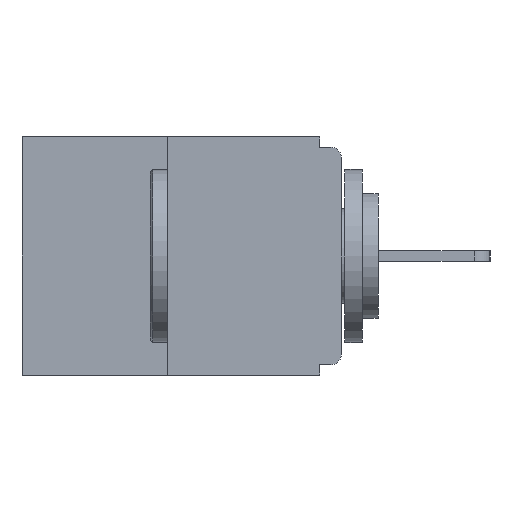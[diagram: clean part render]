
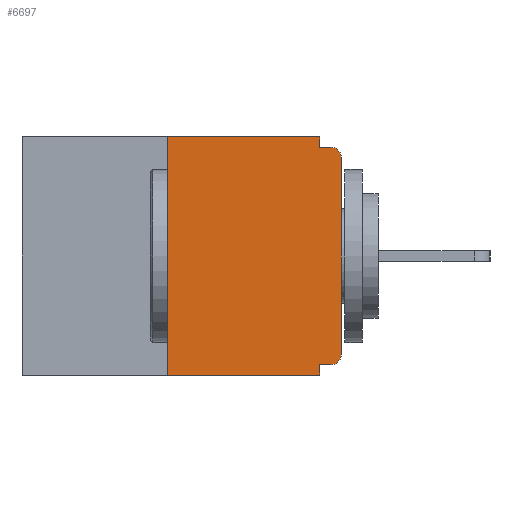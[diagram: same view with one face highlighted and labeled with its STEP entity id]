
A CAD part, left-side view. The second image highlights one B-rep face of the part: STEP entity #6697.
In plain terms, the highlighted planar face has unit normal (-1, 0, 0).
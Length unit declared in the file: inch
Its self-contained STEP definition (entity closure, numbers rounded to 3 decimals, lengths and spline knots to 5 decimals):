
#304 = DIRECTION ( 'NONE',  ( 0., 0., -1. ) ) ;
#586 = VERTEX_POINT ( 'NONE', #8508 ) ;
#661 = CARTESIAN_POINT ( 'NONE',  ( 0., 0.015, -0.015 ) ) ;
#724 = ORIENTED_EDGE ( 'NONE', *, *, #22396, .F. ) ;
#886 = DIRECTION ( 'NONE',  ( 0., -1., 0. ) ) ;
#901 = AXIS2_PLACEMENT_3D ( 'NONE', #9115, #12969, #13385 ) ;
#1353 = LINE ( 'NONE', #16869, #15853 ) ;
#2027 = LINE ( 'NONE', #10971, #6311 ) ;
#2299 = CARTESIAN_POINT ( 'NONE',  ( 0., 0.25, -0.343 ) ) ;
#2434 = EDGE_CURVE ( 'NONE', #12994, #24758, #2027, .T. ) ;
#2632 = CARTESIAN_POINT ( 'NONE',  ( 0., 0.031, -0.328 ) ) ;
#2665 = CARTESIAN_POINT ( 'NONE',  ( 0., 0., 0. ) ) ;
#3444 = ORIENTED_EDGE ( 'NONE', *, *, #16783, .F. ) ;
#3770 = DIRECTION ( 'NONE',  ( 0., 1., 0. ) ) ;
#3921 = VECTOR ( 'NONE', #886, 39.37008 ) ;
#4244 = DIRECTION ( 'NONE',  ( 0., 0., 1. ) ) ;
#4893 = LINE ( 'NONE', #13552, #25785 ) ;
#5158 = DIRECTION ( 'NONE',  ( 0., -1., 0. ) ) ;
#5241 = DIRECTION ( 'NONE',  ( -1., 0., 0. ) ) ;
#6208 = CARTESIAN_POINT ( 'NONE',  ( 0., 0., -0.313 ) ) ;
#6311 = VECTOR ( 'NONE', #304, 39.37008 ) ;
#6369 = EDGE_CURVE ( 'NONE', #16720, #7917, #22410, .T. ) ;
#6527 = EDGE_CURVE ( 'NONE', #7917, #12590, #13054, .T. ) ;
#6697 = ADVANCED_FACE ( 'NONE', ( #27108 ), #9185, .F. ) ;
#6981 = AXIS2_PLACEMENT_3D ( 'NONE', #26558, #11588, #18421 ) ;
#7344 = VERTEX_POINT ( 'NONE', #12671 ) ;
#7557 = VECTOR ( 'NONE', #5158, 39.37008 ) ;
#7917 = VERTEX_POINT ( 'NONE', #6208 ) ;
#8429 = VECTOR ( 'NONE', #23970, 39.37008 ) ;
#8457 = ORIENTED_EDGE ( 'NONE', *, *, #2434, .F. ) ;
#8508 = CARTESIAN_POINT ( 'NONE',  ( 0., 0.031, 0. ) ) ;
#8604 = CARTESIAN_POINT ( 'NONE',  ( 0., 0.015, -0.328 ) ) ;
#8798 = AXIS2_PLACEMENT_3D ( 'NONE', #16028, #5241, #22593 ) ;
#9115 = CARTESIAN_POINT ( 'NONE',  ( 0., 0.015, -0.03 ) ) ;
#9185 = PLANE ( 'NONE',  #6981 ) ;
#9304 = ORIENTED_EDGE ( 'NONE', *, *, #6527, .T. ) ;
#9769 = EDGE_CURVE ( 'NONE', #12590, #15881, #27251, .T. ) ;
#10229 = ORIENTED_EDGE ( 'NONE', *, *, #21097, .F. ) ;
#10971 = CARTESIAN_POINT ( 'NONE',  ( 0., 0.031, -0.343 ) ) ;
#11391 = ORIENTED_EDGE ( 'NONE', *, *, #6369, .T. ) ;
#11405 = CARTESIAN_POINT ( 'NONE',  ( 0., 0.031, -0.015 ) ) ;
#11588 = DIRECTION ( 'NONE',  ( 1., 0., 0. ) ) ;
#12364 = DIRECTION ( 'NONE',  ( 0., -1., 0. ) ) ;
#12531 = LINE ( 'NONE', #20929, #18532 ) ;
#12590 = VERTEX_POINT ( 'NONE', #24279 ) ;
#12671 = CARTESIAN_POINT ( 'NONE',  ( 0., 0.25, 0. ) ) ;
#12969 = DIRECTION ( 'NONE',  ( -1., 0., 0. ) ) ;
#12994 = VERTEX_POINT ( 'NONE', #2632 ) ;
#13054 = LINE ( 'NONE', #2665, #27406 ) ;
#13279 = LINE ( 'NONE', #23556, #8429 ) ;
#13340 = EDGE_LOOP ( 'NONE', ( #3444, #724, #14504, #8457, #10229, #11391, #9304, #26432, #17407, #28130 ) ) ;
#13385 = DIRECTION ( 'NONE',  ( 0., 0., -1. ) ) ;
#13552 = CARTESIAN_POINT ( 'NONE',  ( 0., 0., -0.015 ) ) ;
#13953 = LINE ( 'NONE', #15953, #7557 ) ;
#14371 = DIRECTION ( 'NONE',  ( 0., 0., -1. ) ) ;
#14504 = ORIENTED_EDGE ( 'NONE', *, *, #16815, .T. ) ;
#14956 = EDGE_CURVE ( 'NONE', #16762, #15881, #4893, .T. ) ;
#15136 = VERTEX_POINT ( 'NONE', #2299 ) ;
#15853 = VECTOR ( 'NONE', #3770, 39.37008 ) ;
#15881 = VERTEX_POINT ( 'NONE', #661 ) ;
#15953 = CARTESIAN_POINT ( 'NONE',  ( 0., 0.46, -0.343 ) ) ;
#16028 = CARTESIAN_POINT ( 'NONE',  ( 0., 0.015, -0.313 ) ) ;
#16720 = VERTEX_POINT ( 'NONE', #8604 ) ;
#16762 = VERTEX_POINT ( 'NONE', #11405 ) ;
#16783 = EDGE_CURVE ( 'NONE', #7344, #586, #26918, .T. ) ;
#16815 = EDGE_CURVE ( 'NONE', #15136, #24758, #13953, .T. ) ;
#16869 = CARTESIAN_POINT ( 'NONE',  ( 0., 0., -0.328 ) ) ;
#17407 = ORIENTED_EDGE ( 'NONE', *, *, #14956, .F. ) ;
#17788 = CARTESIAN_POINT ( 'NONE',  ( 0., 0.031, -0.343 ) ) ;
#18421 = DIRECTION ( 'NONE',  ( 0., 0., -1. ) ) ;
#18532 = VECTOR ( 'NONE', #14371, 39.37008 ) ;
#20629 = CARTESIAN_POINT ( 'NONE',  ( 0., 0.46, 0. ) ) ;
#20929 = CARTESIAN_POINT ( 'NONE',  ( 0., 0.031, 0. ) ) ;
#21097 = EDGE_CURVE ( 'NONE', #16720, #12994, #1353, .T. ) ;
#22396 = EDGE_CURVE ( 'NONE', #15136, #7344, #13279, .T. ) ;
#22410 = CIRCLE ( 'NONE', #8798, 0.015 ) ;
#22593 = DIRECTION ( 'NONE',  ( 0., 0., -1. ) ) ;
#23556 = CARTESIAN_POINT ( 'NONE',  ( 0., 0.25, 0. ) ) ;
#23970 = DIRECTION ( 'NONE',  ( 0., 0., 1. ) ) ;
#24279 = CARTESIAN_POINT ( 'NONE',  ( 0., 0., -0.03 ) ) ;
#24713 = EDGE_CURVE ( 'NONE', #586, #16762, #12531, .T. ) ;
#24758 = VERTEX_POINT ( 'NONE', #17788 ) ;
#25785 = VECTOR ( 'NONE', #12364, 39.37008 ) ;
#26432 = ORIENTED_EDGE ( 'NONE', *, *, #9769, .T. ) ;
#26558 = CARTESIAN_POINT ( 'NONE',  ( 0., 0.46, 0. ) ) ;
#26918 = LINE ( 'NONE', #20629, #3921 ) ;
#27108 = FACE_OUTER_BOUND ( 'NONE', #13340, .T. ) ;
#27251 = CIRCLE ( 'NONE', #901, 0.015 ) ;
#27406 = VECTOR ( 'NONE', #4244, 39.37008 ) ;
#28130 = ORIENTED_EDGE ( 'NONE', *, *, #24713, .F. ) ;
